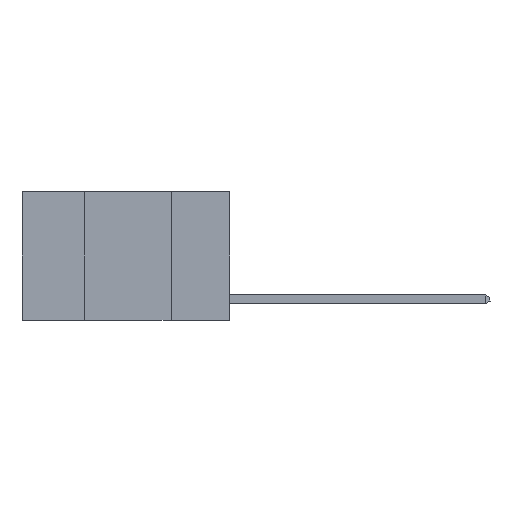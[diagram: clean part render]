
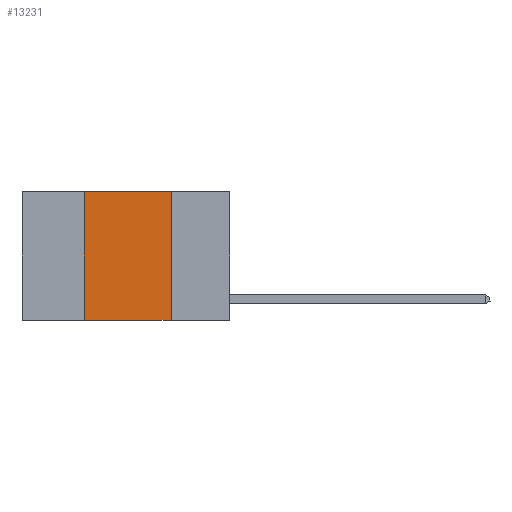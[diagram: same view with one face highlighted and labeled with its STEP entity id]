
A CAD part, left-side view. The second image highlights one B-rep face of the part: STEP entity #13231.
In plain terms, the highlighted planar face has unit normal (-1, 0, 0).
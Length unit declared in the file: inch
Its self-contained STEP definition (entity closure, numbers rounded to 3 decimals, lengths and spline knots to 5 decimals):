
#701 = PLANE ( 'NONE',  #10533 ) ;
#707 = DIRECTION ( 'NONE',  ( 0., 0., 1. ) ) ;
#1520 = DIRECTION ( 'NONE',  ( 0., 0., -1. ) ) ;
#2524 = VERTEX_POINT ( 'NONE', #15499 ) ;
#2624 = DIRECTION ( 'NONE',  ( 1., 0., 0. ) ) ;
#2676 = ORIENTED_EDGE ( 'NONE', *, *, #20316, .T. ) ;
#4444 = VERTEX_POINT ( 'NONE', #18999 ) ;
#4459 = EDGE_CURVE ( 'NONE', #2524, #12761, #4735, .T. ) ;
#4735 = LINE ( 'NONE', #20969, #24312 ) ;
#4751 = VERTEX_POINT ( 'NONE', #13973 ) ;
#8380 = CARTESIAN_POINT ( 'NONE',  ( 0., 0.6, 0. ) ) ;
#8382 = CARTESIAN_POINT ( 'NONE',  ( 0., 0.42, 0. ) ) ;
#8807 = ORIENTED_EDGE ( 'NONE', *, *, #4459, .F. ) ;
#8904 = CARTESIAN_POINT ( 'NONE',  ( 0., 0.6, 0. ) ) ;
#10165 = LINE ( 'NONE', #8904, #15503 ) ;
#10533 = AXIS2_PLACEMENT_3D ( 'NONE', #8380, #2624, #16289 ) ;
#10631 = CARTESIAN_POINT ( 'NONE',  ( 0., 0.17, -0.37 ) ) ;
#10659 = CARTESIAN_POINT ( 'NONE',  ( 0., 0.6, -0.37 ) ) ;
#10851 = DIRECTION ( 'NONE',  ( 0., -1., 0. ) ) ;
#11299 = LINE ( 'NONE', #8382, #21143 ) ;
#12403 = EDGE_LOOP ( 'NONE', ( #8807, #16484, #16016, #2676 ) ) ;
#12761 = VERTEX_POINT ( 'NONE', #10631 ) ;
#13231 = ADVANCED_FACE ( 'NONE', ( #20864 ), #701, .F. ) ;
#13477 = LINE ( 'NONE', #10659, #18145 ) ;
#13973 = CARTESIAN_POINT ( 'NONE',  ( 0., 0.42, 0. ) ) ;
#15499 = CARTESIAN_POINT ( 'NONE',  ( 0., 0.17, 0. ) ) ;
#15503 = VECTOR ( 'NONE', #10851, 39.37008 ) ;
#16016 = ORIENTED_EDGE ( 'NONE', *, *, #22173, .F. ) ;
#16289 = DIRECTION ( 'NONE',  ( 0., 0., -1. ) ) ;
#16484 = ORIENTED_EDGE ( 'NONE', *, *, #24189, .F. ) ;
#18145 = VECTOR ( 'NONE', #22507, 39.37008 ) ;
#18999 = CARTESIAN_POINT ( 'NONE',  ( 0., 0.42, -0.37 ) ) ;
#20316 = EDGE_CURVE ( 'NONE', #4444, #12761, #13477, .T. ) ;
#20864 = FACE_OUTER_BOUND ( 'NONE', #12403, .T. ) ;
#20969 = CARTESIAN_POINT ( 'NONE',  ( 0., 0.17, 0. ) ) ;
#21143 = VECTOR ( 'NONE', #707, 39.37008 ) ;
#22173 = EDGE_CURVE ( 'NONE', #4444, #4751, #11299, .T. ) ;
#22507 = DIRECTION ( 'NONE',  ( 0., -1., 0. ) ) ;
#24189 = EDGE_CURVE ( 'NONE', #4751, #2524, #10165, .T. ) ;
#24312 = VECTOR ( 'NONE', #1520, 39.37008 ) ;
